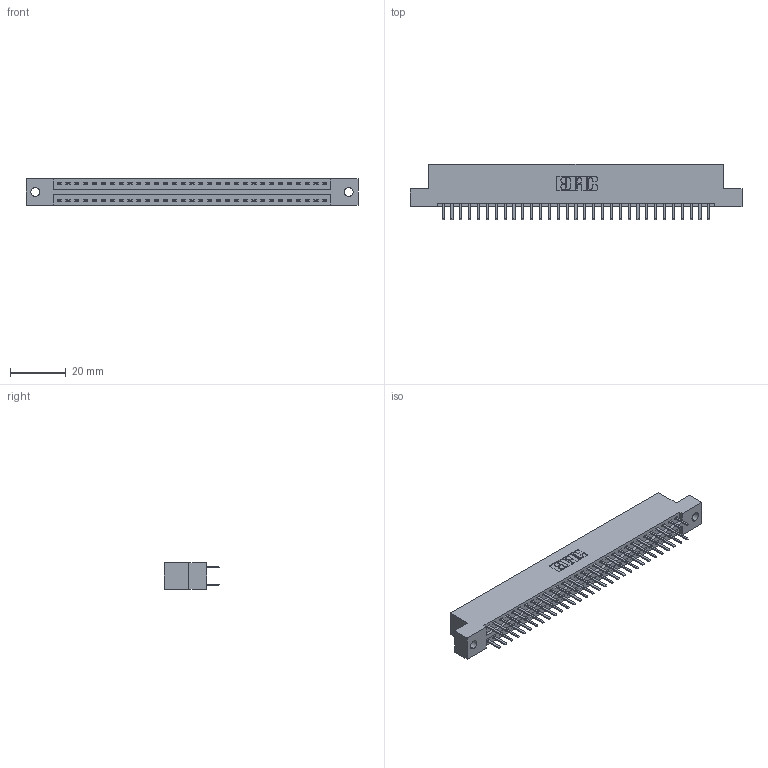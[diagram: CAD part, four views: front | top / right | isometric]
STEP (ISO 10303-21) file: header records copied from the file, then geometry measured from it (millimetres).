
FILE_DESCRIPTION (( 'STEP AP203' ), '1' );
FILE_NAME ('396-062-520-202.STEP', '2019-10-30T16:56:47', ( '' ), ( '' ), 'SwSTEP 2.0', 'SolidWorks 2016', '' );
FILE_SCHEMA (( 'CONFIG_CONTROL_DESIGN' ));
Length unit declared in the file: inch
Products named in the file (3): 346 Part_Flush Mounting Lugs - 0.128 Dia; 345-292-001_345-293-120; 396-062-520-202
Assembly tree (63 placements, depth 2):
  396-062-520-202
    346 Part_Flush Mounting Lugs - 0.128 Dia
    345-292-001_345-293-120  x62
Bounding box: 119 x 20.02 x 9.4 mm (x, y, z)
Volume: 11454.5 mm3; surface area: 15239 mm2
Topology: 63 solids, 63 shells, 3594 faces, 10435 edges, 6790 vertices
Faces by surface type: plane 2370, cylinder 1224
Entity records: 21829 total; most frequent: CARTESIAN_POINT 3624, ORIENTED_EDGE 3546, DIRECTION 3233, EDGE_CURVE 1773, VECTOR 1513, LINE 1513, VERTEX_POINT 1178, AXIS2_PLACEMENT_3D 860
